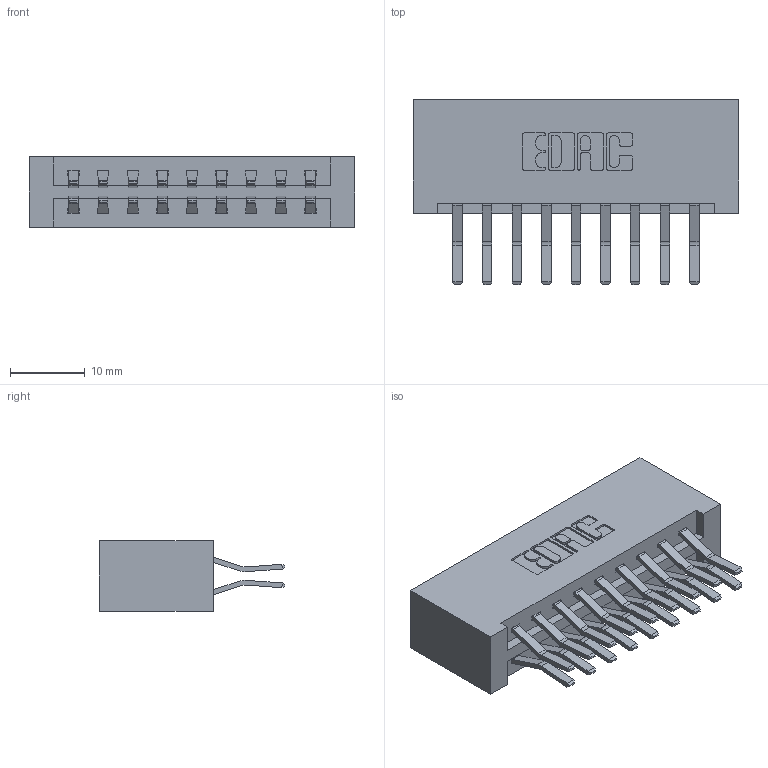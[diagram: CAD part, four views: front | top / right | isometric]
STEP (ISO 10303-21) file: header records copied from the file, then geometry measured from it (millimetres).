
FILE_DESCRIPTION (( 'STEP AP203' ), '1' );
FILE_NAME ('387-018-560-201.STEP', '2018-09-13T02:45:12', ( '' ), ( '' ), 'SwSTEP 2.0', 'SolidWorks 2016', '' );
FILE_SCHEMA (( 'CONFIG_CONTROL_DESIGN' ));
Length unit declared in the file: inch
Products named in the file (3): 345-292-001_560 Tail; 387-018-560-201; 337 Part_No Mounting Lugs
Assembly tree (19 placements, depth 2):
  387-018-560-201
    337 Part_No Mounting Lugs
    345-292-001_560 Tail  x18
Bounding box: 43.54 x 24.78 x 9.4 mm (x, y, z)
Volume: 5027.6 mm3; surface area: 5760.7 mm2
Topology: 19 solids, 19 shells, 1114 faces, 3293 edges, 2170 vertices
Faces by surface type: plane 750, cylinder 364
Entity records: 11057 total; most frequent: CARTESIAN_POINT 1890, ORIENTED_EDGE 1826, DIRECTION 1665, EDGE_CURVE 913, LINE 789, VECTOR 789, VERTEX_POINT 606, AXIS2_PLACEMENT_3D 438
